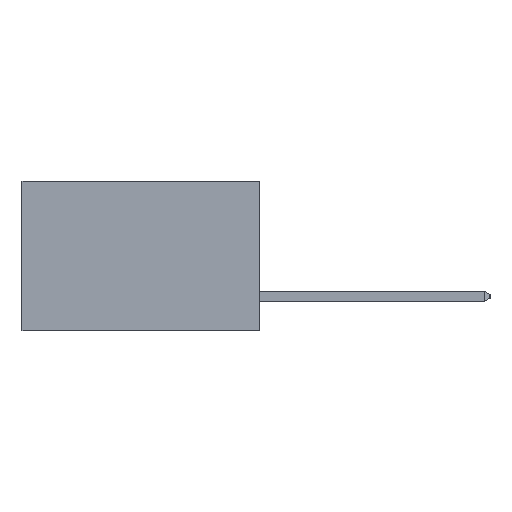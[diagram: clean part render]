
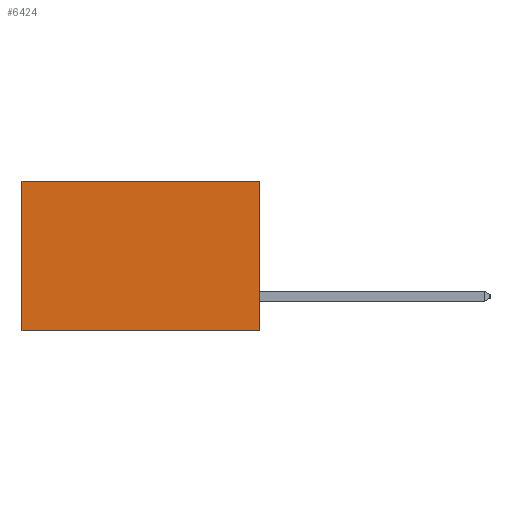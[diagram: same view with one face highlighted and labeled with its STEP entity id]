
A CAD part, left-side view. The second image highlights one B-rep face of the part: STEP entity #6424.
In plain terms, the highlighted planar face has unit normal (-1, 0, 0).
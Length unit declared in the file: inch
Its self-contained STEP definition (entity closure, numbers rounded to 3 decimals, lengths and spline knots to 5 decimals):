
#22 = CARTESIAN_POINT ( 'NONE',  ( 0.277, 0.59, -0.37 ) ) ;
#123 = LINE ( 'NONE', #15751, #5709 ) ;
#1896 = ORIENTED_EDGE ( 'NONE', *, *, #9091, .F. ) ;
#5551 = VERTEX_POINT ( 'NONE', #20866 ) ;
#5709 = VECTOR ( 'NONE', #24686, 39.37008 ) ;
#6424 = ADVANCED_FACE ( 'NONE', ( #26938 ), #16031, .F. ) ;
#6819 = LINE ( 'NONE', #22, #7563 ) ;
#7563 = VECTOR ( 'NONE', #16454, 39.37008 ) ;
#8866 = CARTESIAN_POINT ( 'NONE',  ( 0.277, 0.59, -0.37 ) ) ;
#9091 = EDGE_CURVE ( 'NONE', #5551, #12311, #15591, .T. ) ;
#9442 = CARTESIAN_POINT ( 'NONE',  ( 0.277, 0., -0.37 ) ) ;
#9926 = ORIENTED_EDGE ( 'NONE', *, *, #10278, .T. ) ;
#10278 = EDGE_CURVE ( 'NONE', #5551, #24306, #123, .T. ) ;
#10458 = EDGE_CURVE ( 'NONE', #24306, #16360, #6819, .T. ) ;
#10565 = AXIS2_PLACEMENT_3D ( 'NONE', #14169, #15623, #15593 ) ;
#11283 = VECTOR ( 'NONE', #24831, 39.37008 ) ;
#12311 = VERTEX_POINT ( 'NONE', #13180 ) ;
#12401 = ORIENTED_EDGE ( 'NONE', *, *, #24351, .F. ) ;
#13180 = CARTESIAN_POINT ( 'NONE',  ( 0.277, 0., -0.37 ) ) ;
#14169 = CARTESIAN_POINT ( 'NONE',  ( 0.277, 0., -0.37 ) ) ;
#15591 = LINE ( 'NONE', #9442, #20938 ) ;
#15593 = DIRECTION ( 'NONE',  ( 0., 0., -1. ) ) ;
#15623 = DIRECTION ( 'NONE',  ( 1., 0., 0. ) ) ;
#15751 = CARTESIAN_POINT ( 'NONE',  ( 0.277, 0., 0. ) ) ;
#16031 = PLANE ( 'NONE',  #10565 ) ;
#16261 = ORIENTED_EDGE ( 'NONE', *, *, #10458, .T. ) ;
#16360 = VERTEX_POINT ( 'NONE', #8866 ) ;
#16454 = DIRECTION ( 'NONE',  ( 0., 0., -1. ) ) ;
#18134 = CARTESIAN_POINT ( 'NONE',  ( 0.277, 0., -0.37 ) ) ;
#20866 = CARTESIAN_POINT ( 'NONE',  ( 0.277, 0., 0. ) ) ;
#20938 = VECTOR ( 'NONE', #27505, 39.37008 ) ;
#23360 = LINE ( 'NONE', #18134, #11283 ) ;
#23902 = EDGE_LOOP ( 'NONE', ( #16261, #12401, #1896, #9926 ) ) ;
#24306 = VERTEX_POINT ( 'NONE', #26927 ) ;
#24351 = EDGE_CURVE ( 'NONE', #12311, #16360, #23360, .T. ) ;
#24686 = DIRECTION ( 'NONE',  ( 0., 1., 0. ) ) ;
#24831 = DIRECTION ( 'NONE',  ( 0., 1., 0. ) ) ;
#26927 = CARTESIAN_POINT ( 'NONE',  ( 0.277, 0.59, 0. ) ) ;
#26938 = FACE_OUTER_BOUND ( 'NONE', #23902, .T. ) ;
#27505 = DIRECTION ( 'NONE',  ( 0., 0., -1. ) ) ;
